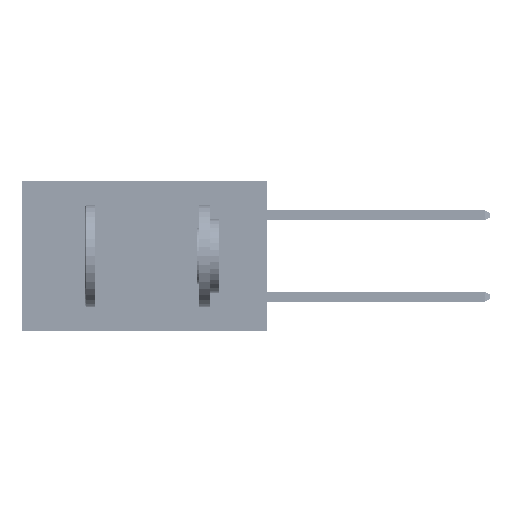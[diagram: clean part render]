
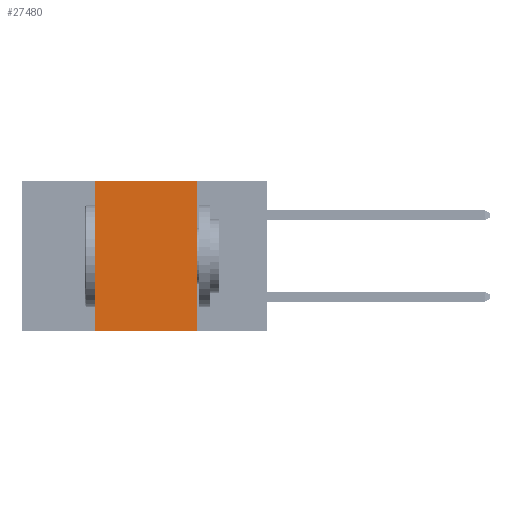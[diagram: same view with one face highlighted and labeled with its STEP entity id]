
A CAD part, left-side view. The second image highlights one B-rep face of the part: STEP entity #27480.
In plain terms, the highlighted planar face has unit normal (-1, 0, 0).
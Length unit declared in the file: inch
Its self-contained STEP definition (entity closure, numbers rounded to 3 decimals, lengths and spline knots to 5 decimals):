
#344 = AXIS2_PLACEMENT_3D ( 'NONE', #35543, #28051, #20736 ) ;
#2336 = EDGE_CURVE ( 'NONE', #31285, #23191, #4730, .T. ) ;
#2402 = CARTESIAN_POINT ( 'NONE',  ( 0., 0.17, 0. ) ) ;
#4592 = CARTESIAN_POINT ( 'NONE',  ( 0., 0.17, -0.37 ) ) ;
#4730 = LINE ( 'NONE', #13149, #46476 ) ;
#7315 = CARTESIAN_POINT ( 'NONE',  ( 0., 0.42, 0. ) ) ;
#8811 = LINE ( 'NONE', #18733, #37965 ) ;
#8959 = PLANE ( 'NONE',  #344 ) ;
#9613 = ORIENTED_EDGE ( 'NONE', *, *, #22894, .F. ) ;
#11773 = DIRECTION ( 'NONE',  ( 0., 0., 1. ) ) ;
#13149 = CARTESIAN_POINT ( 'NONE',  ( 0., 0.6, -0.37 ) ) ;
#14297 = DIRECTION ( 'NONE',  ( 0., -1., 0. ) ) ;
#18511 = CARTESIAN_POINT ( 'NONE',  ( 0., 0.42, -0.37 ) ) ;
#18733 = CARTESIAN_POINT ( 'NONE',  ( 0., 0.17, 0. ) ) ;
#20736 = DIRECTION ( 'NONE',  ( 0., 0., -1. ) ) ;
#22553 = DIRECTION ( 'NONE',  ( 0., 0., -1. ) ) ;
#22894 = EDGE_CURVE ( 'NONE', #31976, #41187, #47222, .T. ) ;
#23191 = VERTEX_POINT ( 'NONE', #4592 ) ;
#23809 = ORIENTED_EDGE ( 'NONE', *, *, #2336, .T. ) ;
#25835 = VECTOR ( 'NONE', #11773, 39.37008 ) ;
#26895 = VECTOR ( 'NONE', #40622, 39.37008 ) ;
#27480 = ADVANCED_FACE ( 'NONE', ( #37706 ), #8959, .F. ) ;
#28051 = DIRECTION ( 'NONE',  ( 1., 0., 0. ) ) ;
#30176 = CARTESIAN_POINT ( 'NONE',  ( 0., 0.42, 0. ) ) ;
#31285 = VERTEX_POINT ( 'NONE', #18511 ) ;
#31976 = VERTEX_POINT ( 'NONE', #7315 ) ;
#35543 = CARTESIAN_POINT ( 'NONE',  ( 0., 0.6, 0. ) ) ;
#36590 = ORIENTED_EDGE ( 'NONE', *, *, #46770, .F. ) ;
#37706 = FACE_OUTER_BOUND ( 'NONE', #48519, .T. ) ;
#37965 = VECTOR ( 'NONE', #22553, 39.37008 ) ;
#40460 = CARTESIAN_POINT ( 'NONE',  ( 0., 0.6, 0. ) ) ;
#40622 = DIRECTION ( 'NONE',  ( 0., -1., 0. ) ) ;
#41049 = EDGE_CURVE ( 'NONE', #31285, #31976, #47345, .T. ) ;
#41187 = VERTEX_POINT ( 'NONE', #2402 ) ;
#45739 = ORIENTED_EDGE ( 'NONE', *, *, #41049, .F. ) ;
#46476 = VECTOR ( 'NONE', #14297, 39.37008 ) ;
#46770 = EDGE_CURVE ( 'NONE', #41187, #23191, #8811, .T. ) ;
#47222 = LINE ( 'NONE', #40460, #26895 ) ;
#47345 = LINE ( 'NONE', #30176, #25835 ) ;
#48519 = EDGE_LOOP ( 'NONE', ( #36590, #9613, #45739, #23809 ) ) ;
